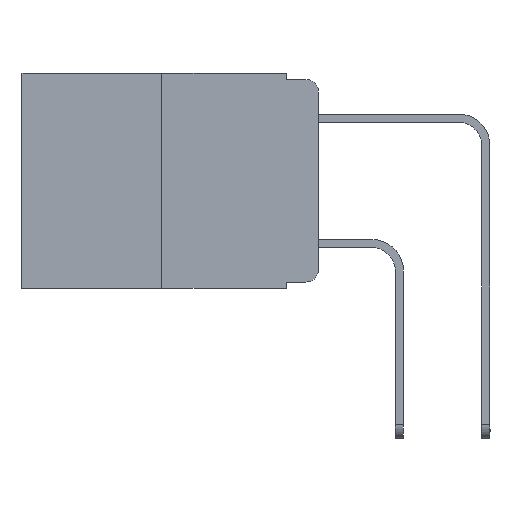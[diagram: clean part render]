
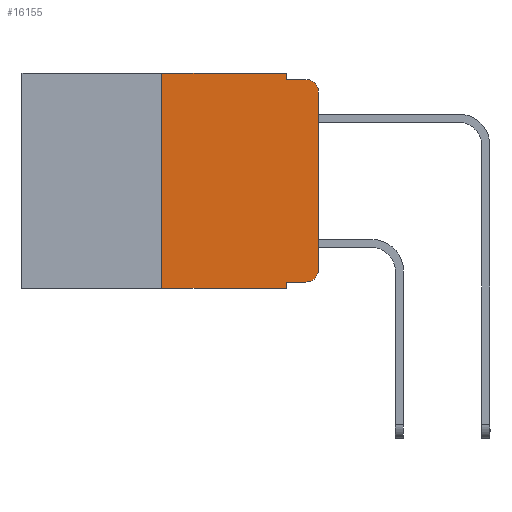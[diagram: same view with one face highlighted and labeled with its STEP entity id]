
A CAD part, left-side view. The second image highlights one B-rep face of the part: STEP entity #16155.
In plain terms, the highlighted planar face has unit normal (-1, 0, 0).
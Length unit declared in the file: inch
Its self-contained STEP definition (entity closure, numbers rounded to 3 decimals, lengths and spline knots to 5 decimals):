
#144 = EDGE_CURVE ( 'NONE', #15277, #3572, #21295, .T. ) ;
#213 = CARTESIAN_POINT ( 'NONE',  ( 0., 0.051, -0.333 ) ) ;
#295 = CARTESIAN_POINT ( 'NONE',  ( 0., 0., -0.03 ) ) ;
#500 = CARTESIAN_POINT ( 'NONE',  ( 0., 0.473, 0. ) ) ;
#674 = VECTOR ( 'NONE', #22615, 39.37008 ) ;
#748 = CARTESIAN_POINT ( 'NONE',  ( 0., 0.473, 0. ) ) ;
#855 = VECTOR ( 'NONE', #12605, 39.37008 ) ;
#916 = ORIENTED_EDGE ( 'NONE', *, *, #1095, .F. ) ;
#1095 = EDGE_CURVE ( 'NONE', #11463, #3765, #8242, .T. ) ;
#1344 = CARTESIAN_POINT ( 'NONE',  ( 0., 0.02, -0.333 ) ) ;
#1666 = CARTESIAN_POINT ( 'NONE',  ( 0., 0.051, -0.01 ) ) ;
#1953 = VECTOR ( 'NONE', #6520, 39.37008 ) ;
#2938 = VERTEX_POINT ( 'NONE', #295 ) ;
#3433 = VECTOR ( 'NONE', #7765, 39.37008 ) ;
#3543 = ORIENTED_EDGE ( 'NONE', *, *, #10566, .T. ) ;
#3572 = VERTEX_POINT ( 'NONE', #16560 ) ;
#3765 = VERTEX_POINT ( 'NONE', #19019 ) ;
#3953 = EDGE_CURVE ( 'NONE', #10102, #6928, #21122, .T. ) ;
#4682 = ORIENTED_EDGE ( 'NONE', *, *, #9070, .F. ) ;
#4691 = CARTESIAN_POINT ( 'NONE',  ( 0., 0.25, 0. ) ) ;
#5379 = AXIS2_PLACEMENT_3D ( 'NONE', #500, #20576, #17124 ) ;
#6104 = PLANE ( 'NONE',  #5379 ) ;
#6217 = CARTESIAN_POINT ( 'NONE',  ( 0., 0.25, -0.343 ) ) ;
#6469 = DIRECTION ( 'NONE',  ( 0., 0., -1. ) ) ;
#6520 = DIRECTION ( 'NONE',  ( 0., 0., 1. ) ) ;
#6928 = VERTEX_POINT ( 'NONE', #7141 ) ;
#6962 = VECTOR ( 'NONE', #17913, 39.37008 ) ;
#7085 = CARTESIAN_POINT ( 'NONE',  ( 0., 0., 0. ) ) ;
#7141 = CARTESIAN_POINT ( 'NONE',  ( 0., 0.051, -0.343 ) ) ;
#7765 = DIRECTION ( 'NONE',  ( 0., -1., 0. ) ) ;
#8242 = LINE ( 'NONE', #748, #3433 ) ;
#8542 = AXIS2_PLACEMENT_3D ( 'NONE', #13515, #11528, #6469 ) ;
#8627 = CARTESIAN_POINT ( 'NONE',  ( 0., 0.051, 0. ) ) ;
#8671 = DIRECTION ( 'NONE',  ( 0., 0., 1. ) ) ;
#8746 = LINE ( 'NONE', #213, #21792 ) ;
#9070 = EDGE_CURVE ( 'NONE', #15645, #6928, #20289, .T. ) ;
#10102 = VERTEX_POINT ( 'NONE', #6217 ) ;
#10452 = DIRECTION ( 'NONE',  ( 0., 0., -1. ) ) ;
#10566 = EDGE_CURVE ( 'NONE', #2938, #3572, #15145, .T. ) ;
#11463 = VERTEX_POINT ( 'NONE', #12323 ) ;
#11528 = DIRECTION ( 'NONE',  ( -1., 0., 0. ) ) ;
#12089 = FACE_OUTER_BOUND ( 'NONE', #19005, .T. ) ;
#12323 = CARTESIAN_POINT ( 'NONE',  ( 0., 0.25, 0. ) ) ;
#12420 = EDGE_CURVE ( 'NONE', #16701, #2938, #18507, .T. ) ;
#12605 = DIRECTION ( 'NONE',  ( 0., -1., 0. ) ) ;
#13515 = CARTESIAN_POINT ( 'NONE',  ( 0., 0.02, -0.313 ) ) ;
#14425 = CARTESIAN_POINT ( 'NONE',  ( 0., 0.051, -0.01 ) ) ;
#14506 = CARTESIAN_POINT ( 'NONE',  ( 0., 0.02, -0.03 ) ) ;
#14820 = AXIS2_PLACEMENT_3D ( 'NONE', #14506, #19567, #19731 ) ;
#15016 = ORIENTED_EDGE ( 'NONE', *, *, #16410, .F. ) ;
#15145 = CIRCLE ( 'NONE', #14820, 0.02 ) ;
#15277 = VERTEX_POINT ( 'NONE', #1666 ) ;
#15486 = CARTESIAN_POINT ( 'NONE',  ( 0., 0.051, -0.333 ) ) ;
#15645 = VERTEX_POINT ( 'NONE', #15486 ) ;
#16155 = ADVANCED_FACE ( 'NONE', ( #12089 ), #6104, .F. ) ;
#16230 = ORIENTED_EDGE ( 'NONE', *, *, #144, .F. ) ;
#16410 = EDGE_CURVE ( 'NONE', #3765, #15277, #21406, .T. ) ;
#16560 = CARTESIAN_POINT ( 'NONE',  ( 0., 0.02, -0.01 ) ) ;
#16701 = VERTEX_POINT ( 'NONE', #16703 ) ;
#16703 = CARTESIAN_POINT ( 'NONE',  ( 0., 0., -0.313 ) ) ;
#16842 = EDGE_CURVE ( 'NONE', #17015, #16701, #21873, .T. ) ;
#17015 = VERTEX_POINT ( 'NONE', #1344 ) ;
#17124 = DIRECTION ( 'NONE',  ( 0., 0., -1. ) ) ;
#17279 = ORIENTED_EDGE ( 'NONE', *, *, #3953, .T. ) ;
#17529 = ORIENTED_EDGE ( 'NONE', *, *, #17612, .F. ) ;
#17612 = EDGE_CURVE ( 'NONE', #10102, #11463, #20132, .T. ) ;
#17781 = CARTESIAN_POINT ( 'NONE',  ( 0., 0.051, 0. ) ) ;
#17913 = DIRECTION ( 'NONE',  ( 0., 0., -1. ) ) ;
#17956 = VECTOR ( 'NONE', #8671, 39.37008 ) ;
#18290 = EDGE_CURVE ( 'NONE', #15645, #17015, #8746, .T. ) ;
#18507 = LINE ( 'NONE', #7085, #17956 ) ;
#19005 = EDGE_LOOP ( 'NONE', ( #21556, #3543, #16230, #15016, #916, #17529, #17279, #4682, #22749, #21075 ) ) ;
#19019 = CARTESIAN_POINT ( 'NONE',  ( 0., 0.051, 0. ) ) ;
#19567 = DIRECTION ( 'NONE',  ( -1., 0., 0. ) ) ;
#19731 = DIRECTION ( 'NONE',  ( 0., 0., -1. ) ) ;
#20132 = LINE ( 'NONE', #4691, #1953 ) ;
#20289 = LINE ( 'NONE', #17781, #20843 ) ;
#20306 = DIRECTION ( 'NONE',  ( 0., -1., 0. ) ) ;
#20576 = DIRECTION ( 'NONE',  ( 1., 0., 0. ) ) ;
#20719 = CARTESIAN_POINT ( 'NONE',  ( 0., 0.473, -0.343 ) ) ;
#20843 = VECTOR ( 'NONE', #10452, 39.37008 ) ;
#21075 = ORIENTED_EDGE ( 'NONE', *, *, #16842, .T. ) ;
#21122 = LINE ( 'NONE', #20719, #674 ) ;
#21295 = LINE ( 'NONE', #14425, #855 ) ;
#21406 = LINE ( 'NONE', #8627, #6962 ) ;
#21556 = ORIENTED_EDGE ( 'NONE', *, *, #12420, .T. ) ;
#21792 = VECTOR ( 'NONE', #20306, 39.37008 ) ;
#21873 = CIRCLE ( 'NONE', #8542, 0.02 ) ;
#22615 = DIRECTION ( 'NONE',  ( 0., -1., 0. ) ) ;
#22749 = ORIENTED_EDGE ( 'NONE', *, *, #18290, .T. ) ;
